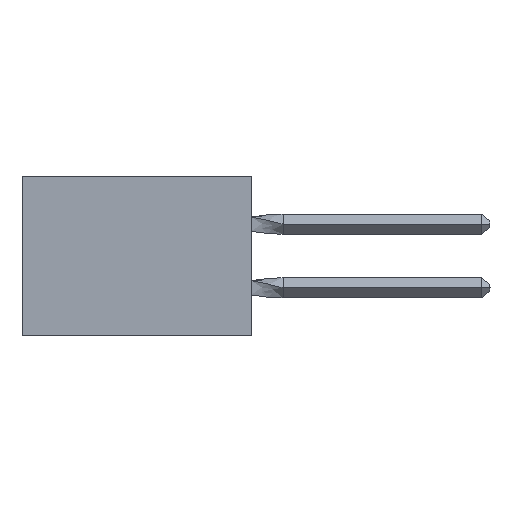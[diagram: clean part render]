
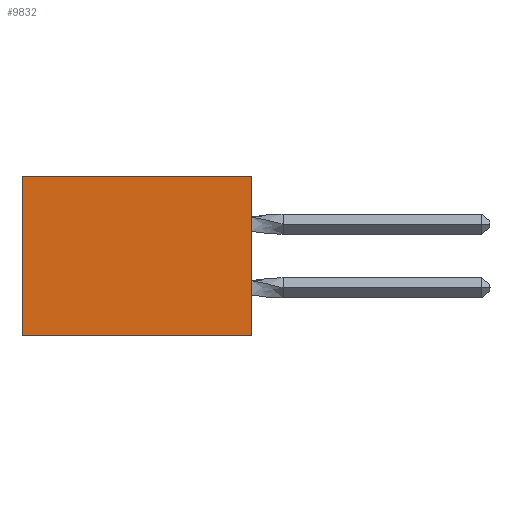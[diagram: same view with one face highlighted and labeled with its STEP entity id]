
A CAD part, left-side view. The second image highlights one B-rep face of the part: STEP entity #9832.
In plain terms, the highlighted planar face has unit normal (-1, 0, 0).
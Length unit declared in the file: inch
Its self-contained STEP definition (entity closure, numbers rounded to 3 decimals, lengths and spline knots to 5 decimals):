
#1355 = CARTESIAN_POINT ( 'NONE',  ( 0.305, 0.72, 0. ) ) ;
#1687 = CARTESIAN_POINT ( 'NONE',  ( 0.305, 0.72, -0.5 ) ) ;
#1764 = VECTOR ( 'NONE', #21488, 39.37008 ) ;
#2191 = LINE ( 'NONE', #1687, #11629 ) ;
#2336 = ORIENTED_EDGE ( 'NONE', *, *, #18120, .F. ) ;
#2516 = VECTOR ( 'NONE', #3174, 39.37008 ) ;
#3174 = DIRECTION ( 'NONE',  ( 0., 1., 0. ) ) ;
#3442 = EDGE_CURVE ( 'NONE', #18870, #15991, #23150, .T. ) ;
#3718 = ORIENTED_EDGE ( 'NONE', *, *, #23427, .F. ) ;
#8285 = VERTEX_POINT ( 'NONE', #23119 ) ;
#8581 = VECTOR ( 'NONE', #12077, 39.37008 ) ;
#9832 = ADVANCED_FACE ( 'NONE', ( #21029 ), #17610, .F. ) ;
#10321 = DIRECTION ( 'NONE',  ( 1., 0., 0. ) ) ;
#11629 = VECTOR ( 'NONE', #14504, 39.37008 ) ;
#11703 = VERTEX_POINT ( 'NONE', #14474 ) ;
#12077 = DIRECTION ( 'NONE',  ( 0., 0., -1. ) ) ;
#12274 = CARTESIAN_POINT ( 'NONE',  ( 0.305, 0., -0.5 ) ) ;
#12297 = DIRECTION ( 'NONE',  ( 0., 0., -1. ) ) ;
#13615 = CARTESIAN_POINT ( 'NONE',  ( 0.305, 0., 0. ) ) ;
#14155 = CARTESIAN_POINT ( 'NONE',  ( 0.305, 0., 0. ) ) ;
#14238 = CARTESIAN_POINT ( 'NONE',  ( 0.305, 0., -0.5 ) ) ;
#14474 = CARTESIAN_POINT ( 'NONE',  ( 0.305, 0.72, -0.5 ) ) ;
#14504 = DIRECTION ( 'NONE',  ( 0., 0., -1. ) ) ;
#15171 = EDGE_CURVE ( 'NONE', #15991, #11703, #2191, .T. ) ;
#15511 = ORIENTED_EDGE ( 'NONE', *, *, #3442, .T. ) ;
#15991 = VERTEX_POINT ( 'NONE', #1355 ) ;
#17502 = LINE ( 'NONE', #14238, #8581 ) ;
#17610 = PLANE ( 'NONE',  #23392 ) ;
#17754 = EDGE_LOOP ( 'NONE', ( #19405, #2336, #3718, #15511 ) ) ;
#18120 = EDGE_CURVE ( 'NONE', #8285, #11703, #20978, .T. ) ;
#18870 = VERTEX_POINT ( 'NONE', #13615 ) ;
#19405 = ORIENTED_EDGE ( 'NONE', *, *, #15171, .T. ) ;
#20978 = LINE ( 'NONE', #12274, #1764 ) ;
#21029 = FACE_OUTER_BOUND ( 'NONE', #17754, .T. ) ;
#21277 = CARTESIAN_POINT ( 'NONE',  ( 0.305, 0., -0.5 ) ) ;
#21488 = DIRECTION ( 'NONE',  ( 0., 1., 0. ) ) ;
#23119 = CARTESIAN_POINT ( 'NONE',  ( 0.305, 0., -0.5 ) ) ;
#23150 = LINE ( 'NONE', #14155, #2516 ) ;
#23392 = AXIS2_PLACEMENT_3D ( 'NONE', #21277, #10321, #12297 ) ;
#23427 = EDGE_CURVE ( 'NONE', #18870, #8285, #17502, .T. ) ;
